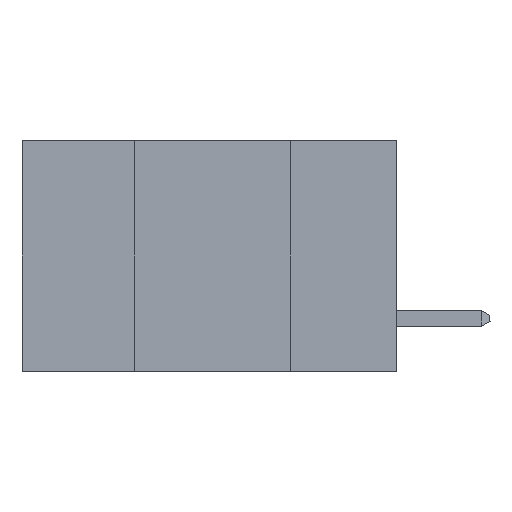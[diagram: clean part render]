
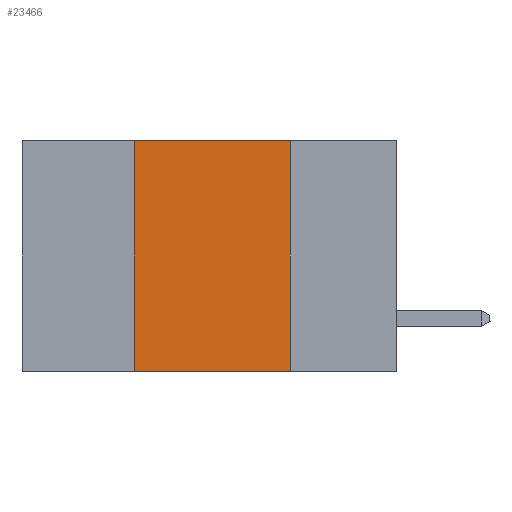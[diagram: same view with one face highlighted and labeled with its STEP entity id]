
A CAD part, left-side view. The second image highlights one B-rep face of the part: STEP entity #23466.
In plain terms, the highlighted planar face has unit normal (-1, 0, 0).
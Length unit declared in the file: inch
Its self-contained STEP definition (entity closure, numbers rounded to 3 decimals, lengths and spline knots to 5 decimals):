
#208 = CARTESIAN_POINT ( 'NONE',  ( 0., 0.17, -0.37 ) ) ;
#1623 = CARTESIAN_POINT ( 'NONE',  ( 0., 0.42, -0.37 ) ) ;
#2974 = LINE ( 'NONE', #20750, #27034 ) ;
#4174 = EDGE_CURVE ( 'NONE', #21507, #9304, #2974, .T. ) ;
#5025 = EDGE_CURVE ( 'NONE', #20751, #21779, #9044, .T. ) ;
#5069 = DIRECTION ( 'NONE',  ( 0., -1., 0. ) ) ;
#5150 = DIRECTION ( 'NONE',  ( 0., 0., -1. ) ) ;
#7388 = CARTESIAN_POINT ( 'NONE',  ( 0., 0.17, 0. ) ) ;
#9044 = LINE ( 'NONE', #18908, #27577 ) ;
#9304 = VERTEX_POINT ( 'NONE', #208 ) ;
#9710 = DIRECTION ( 'NONE',  ( 0., -1., 0. ) ) ;
#11031 = EDGE_LOOP ( 'NONE', ( #25781, #26501, #24638, #13744 ) ) ;
#11509 = PLANE ( 'NONE',  #20894 ) ;
#12115 = FACE_OUTER_BOUND ( 'NONE', #11031, .T. ) ;
#13744 = ORIENTED_EDGE ( 'NONE', *, *, #4174, .T. ) ;
#13862 = DIRECTION ( 'NONE',  ( 1., 0., 0. ) ) ;
#14909 = CARTESIAN_POINT ( 'NONE',  ( 0., 0.42, 0. ) ) ;
#16288 = VECTOR ( 'NONE', #23529, 39.37008 ) ;
#17154 = CARTESIAN_POINT ( 'NONE',  ( 0., 0.17, 0. ) ) ;
#17378 = LINE ( 'NONE', #7388, #22792 ) ;
#18908 = CARTESIAN_POINT ( 'NONE',  ( 0., 0.6, 0. ) ) ;
#20750 = CARTESIAN_POINT ( 'NONE',  ( 0., 0.6, -0.37 ) ) ;
#20751 = VERTEX_POINT ( 'NONE', #14909 ) ;
#20894 = AXIS2_PLACEMENT_3D ( 'NONE', #25329, #13862, #29942 ) ;
#21317 = CARTESIAN_POINT ( 'NONE',  ( 0., 0.42, 0. ) ) ;
#21507 = VERTEX_POINT ( 'NONE', #1623 ) ;
#21779 = VERTEX_POINT ( 'NONE', #17154 ) ;
#22792 = VECTOR ( 'NONE', #5150, 39.37008 ) ;
#23466 = ADVANCED_FACE ( 'NONE', ( #12115 ), #11509, .F. ) ;
#23529 = DIRECTION ( 'NONE',  ( 0., 0., 1. ) ) ;
#24638 = ORIENTED_EDGE ( 'NONE', *, *, #28090, .F. ) ;
#25329 = CARTESIAN_POINT ( 'NONE',  ( 0., 0.6, 0. ) ) ;
#25781 = ORIENTED_EDGE ( 'NONE', *, *, #26551, .F. ) ;
#26501 = ORIENTED_EDGE ( 'NONE', *, *, #5025, .F. ) ;
#26551 = EDGE_CURVE ( 'NONE', #21779, #9304, #17378, .T. ) ;
#27034 = VECTOR ( 'NONE', #5069, 39.37008 ) ;
#27577 = VECTOR ( 'NONE', #9710, 39.37008 ) ;
#28090 = EDGE_CURVE ( 'NONE', #21507, #20751, #28482, .T. ) ;
#28482 = LINE ( 'NONE', #21317, #16288 ) ;
#29942 = DIRECTION ( 'NONE',  ( 0., 0., -1. ) ) ;
